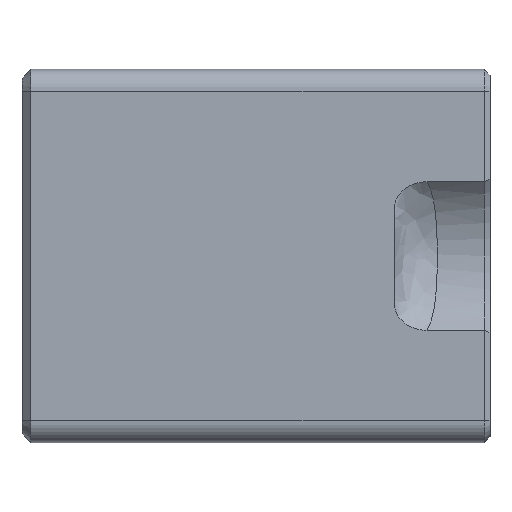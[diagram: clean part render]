
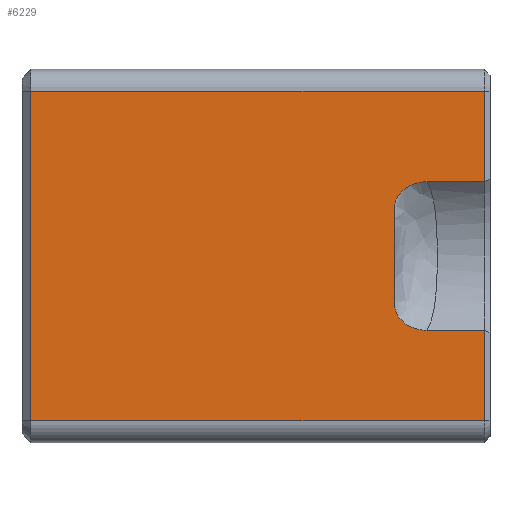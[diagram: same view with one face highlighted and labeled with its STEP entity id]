
A CAD part, front view. The second image highlights one B-rep face of the part: STEP entity #6229.
In plain terms, the highlighted planar face has unit normal (0, -1, 0).
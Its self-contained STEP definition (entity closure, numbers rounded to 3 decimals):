
#620=B_SPLINE_CURVE_WITH_KNOTS('',3,(#15276,#15277,#15278,#15279,#15280,
#15281,#15282,#15283,#15284,#15285,#15286,#15287,#15288,#15289,#15290,#15291,
#15292,#15293,#15294,#15295),.UNSPECIFIED.,.F.,.F.,(4,2,2,2,2,2,2,2,2,4),
(0.,0.,0.,0.002,0.007,
0.018,0.04,0.085,0.157,
0.234),.UNSPECIFIED.);
#621=B_SPLINE_CURVE_WITH_KNOTS('',3,(#15299,#15300,#15301,#15302,#15303,
#15304,#15305,#15306,#15307,#15308,#15309,#15310,#15311,#15312,#15313,#15314,
#15315,#15316,#15317,#15318),.UNSPECIFIED.,.F.,.F.,(4,2,2,2,2,2,2,2,2,4),
(0.,0.102,0.197,0.257,0.286,
0.3,0.306,0.31,0.31,
0.31),.UNSPECIFIED.);
#750=PLANE('',#6722);
#1176=FACE_OUTER_BOUND('',#1575,.T.);
#1575=EDGE_LOOP('',(#5610,#5611,#5612,#5613,#5614,#5615,#5616,#5617,#5618,
#5619));
#1875=LINE('',#15243,#2168);
#1884=LINE('',#15265,#2177);
#1885=LINE('',#15270,#2178);
#1886=LINE('',#15274,#2179);
#1887=LINE('',#15297,#2180);
#1888=LINE('',#15319,#2181);
#1889=LINE('',#15321,#2182);
#1890=LINE('',#15322,#2183);
#2168=VECTOR('',#7804,10.);
#2177=VECTOR('',#7837,10.);
#2178=VECTOR('',#7844,10.);
#2179=VECTOR('',#7849,10.);
#2180=VECTOR('',#7850,10.);
#2181=VECTOR('',#7851,10.);
#2182=VECTOR('',#7852,10.);
#2183=VECTOR('',#7853,10.);
#2973=VERTEX_POINT('',#15230);
#2974=VERTEX_POINT('',#15235);
#2975=VERTEX_POINT('',#15242);
#2976=VERTEX_POINT('',#15261);
#2977=VERTEX_POINT('',#15269);
#2978=VERTEX_POINT('',#15273);
#2979=VERTEX_POINT('',#15275);
#2980=VERTEX_POINT('',#15296);
#2981=VERTEX_POINT('',#15298);
#2982=VERTEX_POINT('',#15320);
#3853=EDGE_CURVE('',#2974,#2975,#1875,.T.);
#3866=EDGE_CURVE('',#2976,#2973,#1884,.T.);
#3868=EDGE_CURVE('',#2975,#2977,#1885,.T.);
#3870=EDGE_CURVE('',#2974,#2978,#1886,.T.);
#3871=EDGE_CURVE('',#2979,#2978,#620,.T.);
#3872=EDGE_CURVE('',#2979,#2980,#1887,.T.);
#3873=EDGE_CURVE('',#2980,#2981,#621,.F.);
#3874=EDGE_CURVE('',#2981,#2973,#1888,.T.);
#3875=EDGE_CURVE('',#2982,#2976,#1889,.T.);
#3876=EDGE_CURVE('',#2977,#2982,#1890,.T.);
#5610=ORIENTED_EDGE('',*,*,#3853,.F.);
#5611=ORIENTED_EDGE('',*,*,#3870,.T.);
#5612=ORIENTED_EDGE('',*,*,#3871,.F.);
#5613=ORIENTED_EDGE('',*,*,#3872,.T.);
#5614=ORIENTED_EDGE('',*,*,#3873,.T.);
#5615=ORIENTED_EDGE('',*,*,#3874,.T.);
#5616=ORIENTED_EDGE('',*,*,#3866,.F.);
#5617=ORIENTED_EDGE('',*,*,#3875,.F.);
#5618=ORIENTED_EDGE('',*,*,#3876,.F.);
#5619=ORIENTED_EDGE('',*,*,#3868,.F.);
#6229=ADVANCED_FACE('',(#1176),#750,.T.);
#6722=AXIS2_PLACEMENT_3D('',#15272,#7847,#7848);
#7804=DIRECTION('',(0.,0.,-1.));
#7837=DIRECTION('',(0.,0.,-1.));
#7844=DIRECTION('',(-1.,0.,0.));
#7847=DIRECTION('center_axis',(0.,-1.,0.));
#7848=DIRECTION('ref_axis',(0.,0.,1.));
#7849=DIRECTION('',(-1.,0.,0.));
#7850=DIRECTION('',(0.,0.,1.));
#7851=DIRECTION('',(1.,0.,0.));
#7852=DIRECTION('',(1.,0.,0.));
#7853=DIRECTION('',(0.,0.,1.));
#15230=CARTESIAN_POINT('',(-183.534,-11.455,5.083));
#15235=CARTESIAN_POINT('',(-183.534,-11.455,-5.083));
#15242=CARTESIAN_POINT('',(-183.534,-11.455,-11.264));
#15243=CARTESIAN_POINT('',(-183.534,-11.455,-6.128));
#15261=CARTESIAN_POINT('',(-183.534,-11.455,11.264));
#15265=CARTESIAN_POINT('',(-183.534,-11.455,-6.128));
#15269=CARTESIAN_POINT('',(-214.534,-11.455,-11.264));
#15270=CARTESIAN_POINT('',(-183.134,-11.455,-11.264));
#15272=CARTESIAN_POINT('Origin',(-183.134,-11.455,-12.256));
#15273=CARTESIAN_POINT('',(-187.44,-11.455,-5.083));
#15274=CARTESIAN_POINT('',(-183.134,-11.455,-5.083));
#15275=CARTESIAN_POINT('',(-189.634,-11.455,-3.546));
#15276=CARTESIAN_POINT('Ctrl Pts',(-189.634,-11.455,-3.546));
#15277=CARTESIAN_POINT('Ctrl Pts',(-189.634,-11.455,-3.546));
#15278=CARTESIAN_POINT('Ctrl Pts',(-189.634,-11.455,-3.547));
#15279=CARTESIAN_POINT('Ctrl Pts',(-189.634,-11.455,-3.548));
#15280=CARTESIAN_POINT('Ctrl Pts',(-189.634,-11.455,-3.549));
#15281=CARTESIAN_POINT('Ctrl Pts',(-189.634,-11.455,-3.558));
#15282=CARTESIAN_POINT('Ctrl Pts',(-189.633,-11.455,-3.566));
#15283=CARTESIAN_POINT('Ctrl Pts',(-189.63,-11.455,-3.592));
#15284=CARTESIAN_POINT('Ctrl Pts',(-189.627,-11.455,-3.61));
#15285=CARTESIAN_POINT('Ctrl Pts',(-189.616,-11.455,-3.667));
#15286=CARTESIAN_POINT('Ctrl Pts',(-189.605,-11.455,-3.707));
#15287=CARTESIAN_POINT('Ctrl Pts',(-189.566,-11.455,-3.826));
#15288=CARTESIAN_POINT('Ctrl Pts',(-189.531,-11.455,-3.905));
#15289=CARTESIAN_POINT('Ctrl Pts',(-189.407,-11.455,-4.136));
#15290=CARTESIAN_POINT('Ctrl Pts',(-189.297,-11.455,
-4.279));
#15291=CARTESIAN_POINT('Ctrl Pts',(-188.973,-11.455,
-4.603));
#15292=CARTESIAN_POINT('Ctrl Pts',(-188.724,-11.455,-4.771));
#15293=CARTESIAN_POINT('Ctrl Pts',(-188.119,-11.455,-5.02));
#15294=CARTESIAN_POINT('Ctrl Pts',(-187.781,-11.455,-5.083));
#15295=CARTESIAN_POINT('Ctrl Pts',(-187.44,-11.455,-5.083));
#15296=CARTESIAN_POINT('',(-189.634,-11.455,3.546));
#15297=CARTESIAN_POINT('',(-189.634,-11.455,-6.128));
#15298=CARTESIAN_POINT('',(-187.44,-11.455,5.083));
#15299=CARTESIAN_POINT('Ctrl Pts',(-187.44,-11.455,5.083));
#15300=CARTESIAN_POINT('Ctrl Pts',(-187.781,-11.455,5.083));
#15301=CARTESIAN_POINT('Ctrl Pts',(-188.119,-11.455,5.02));
#15302=CARTESIAN_POINT('Ctrl Pts',(-188.724,-11.455,4.771));
#15303=CARTESIAN_POINT('Ctrl Pts',(-188.973,-11.455,
4.603));
#15304=CARTESIAN_POINT('Ctrl Pts',(-189.297,-11.455,
4.279));
#15305=CARTESIAN_POINT('Ctrl Pts',(-189.407,-11.455,4.136));
#15306=CARTESIAN_POINT('Ctrl Pts',(-189.531,-11.455,3.905));
#15307=CARTESIAN_POINT('Ctrl Pts',(-189.566,-11.455,3.826));
#15308=CARTESIAN_POINT('Ctrl Pts',(-189.605,-11.455,3.707));
#15309=CARTESIAN_POINT('Ctrl Pts',(-189.616,-11.455,3.667));
#15310=CARTESIAN_POINT('Ctrl Pts',(-189.627,-11.455,3.61));
#15311=CARTESIAN_POINT('Ctrl Pts',(-189.63,-11.455,3.592));
#15312=CARTESIAN_POINT('Ctrl Pts',(-189.633,-11.455,3.565));
#15313=CARTESIAN_POINT('Ctrl Pts',(-189.634,-11.455,3.557));
#15314=CARTESIAN_POINT('Ctrl Pts',(-189.634,-11.455,3.549));
#15315=CARTESIAN_POINT('Ctrl Pts',(-189.634,-11.455,3.548));
#15316=CARTESIAN_POINT('Ctrl Pts',(-189.634,-11.455,3.547));
#15317=CARTESIAN_POINT('Ctrl Pts',(-189.634,-11.455,3.546));
#15318=CARTESIAN_POINT('Ctrl Pts',(-189.634,-11.455,3.546));
#15319=CARTESIAN_POINT('',(-183.134,-11.455,5.083));
#15320=CARTESIAN_POINT('',(-214.534,-11.455,11.264));
#15321=CARTESIAN_POINT('',(-183.134,-11.455,11.264));
#15322=CARTESIAN_POINT('',(-214.534,-11.455,-6.128));
